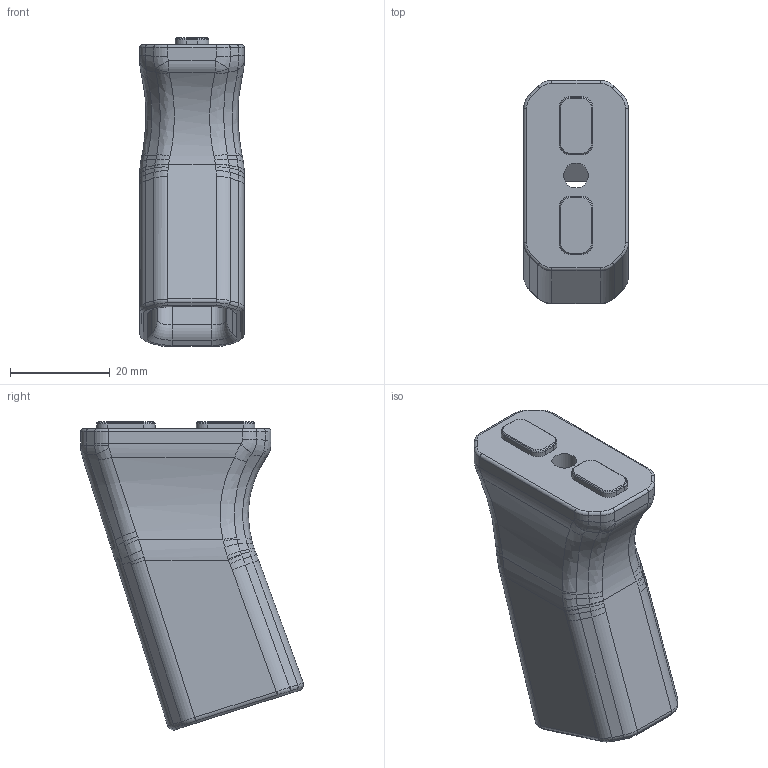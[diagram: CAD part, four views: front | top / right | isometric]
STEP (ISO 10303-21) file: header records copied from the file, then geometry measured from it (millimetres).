
FILE_DESCRIPTION(/* description */ (''),/* implementation_level */ '2;1');
FILE_NAME(/* name */ 'Standard.step',/* time_stamp */ '2021-11-24T02:39:30-05:00',/* author */ (''),/* organization */ (''),/* preprocessor_version */ 'ST-DEVELOPER v18.1',/* originating_system */ 'Autodesk Translation Framework v10.10.0.1391',/* authorisation */ '');
FILE_SCHEMA (('AUTOMOTIVE_DESIGN { 1 0 10303 214 3 1 1 }'));
Length unit declared in the file: millimetre
Products named in the file (1): Standard
Bounding box: 21 x 44.72 x 61.96 mm (x, y, z)
Volume: 17910.4 mm3; surface area: 10187.4 mm2
Topology: 1 solids, 1 shells, 345 faces, 799 edges, 460 vertices
Faces by surface type: bspline 165, cylinder 76, plane 58, torus 30, cone 14, sphere 2
Full cylindrical faces by diameter (mm): 5 x1, 13.416 x1
Entity records: 13001 total; most frequent: CARTESIAN_POINT 6016, ORIENTED_EDGE 1590, DIRECTION 1188, EDGE_CURVE 795, AXIS2_PLACEMENT_3D 473, VERTEX_POINT 460, EDGE_LOOP 355, FACE_OUTER_BOUND 345
